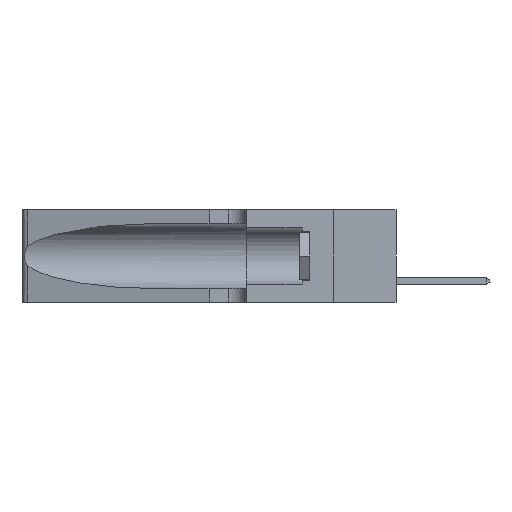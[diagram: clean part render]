
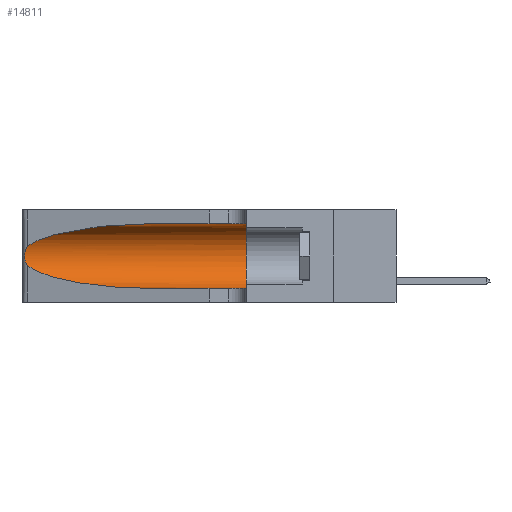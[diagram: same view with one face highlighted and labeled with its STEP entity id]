
A CAD part, left-side view. The second image highlights one B-rep face of the part: STEP entity #14811.
In plain terms, the highlighted cylindrical face has radius 3.308 mm (diameter 6.617 mm), a partial arc.
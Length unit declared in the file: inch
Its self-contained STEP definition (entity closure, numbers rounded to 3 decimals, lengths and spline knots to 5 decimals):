
#454 = EDGE_CURVE ( 'NONE', #9702, #13073, #2145, .T. ) ;
#781 = CARTESIAN_POINT ( 'NONE',  ( 0.1305, 0.72297, 0.31525 ) ) ;
#1479 = CARTESIAN_POINT ( 'NONE',  ( 0.1305, 1.61858, 0.31525 ) ) ;
#2141 = CARTESIAN_POINT ( 'NONE',  ( 0.25856, 1.23593, 0.16098 ) ) ;
#2145 =( BOUNDED_CURVE ( )  B_SPLINE_CURVE ( 3, ( #781, #26645, #13333, #13457 ),
 .UNSPECIFIED., .F., .T. ) 
 B_SPLINE_CURVE_WITH_KNOTS ( ( 4, 4 ),
 ( 1.5708, 2.84003 ),
 .UNSPECIFIED. ) 
 CURVE ( )  GEOMETRIC_REPRESENTATION_ITEM ( )  RATIONAL_B_SPLINE_CURVE ( ( 1., 0.87, 0.87, 1. ) ) 
 REPRESENTATION_ITEM ( '' )  );
#2246 = CARTESIAN_POINT ( 'NONE',  ( 0.25639, 1.23184, 0.21858 ) ) ;
#2332 = B_SPLINE_CURVE_WITH_KNOTS ( 'NONE', 3,
 ( #25720, #20434, #2246, #20649, #7427, #25504, #9921, #10036, #7210, #2141, #9804, #23312, #28381, #4944 ),
 .UNSPECIFIED., .F., .F.,
 ( 4, 2, 2, 2, 2, 2, 4 ),
 ( 0., 0.00027, 0.00053, 0.00107, 0.0016, 0.00187, 0.00214 ),
 .UNSPECIFIED. ) ;
#4106 = VERTEX_POINT ( 'NONE', #18051 ) ;
#4324 = VERTEX_POINT ( 'NONE', #7774 ) ;
#4944 = CARTESIAN_POINT ( 'NONE',  ( 0.25487, 1.22718, 0.14631 ) ) ;
#7031 = ORIENTED_EDGE ( 'NONE', *, *, #20623, .T. ) ;
#7078 = CARTESIAN_POINT ( 'NONE',  ( 0.1305, 1.61858, 0.05475 ) ) ;
#7210 = CARTESIAN_POINT ( 'NONE',  ( 0.26017, 1.23833, 0.17102 ) ) ;
#7427 = CARTESIAN_POINT ( 'NONE',  ( 0.25854, 1.2359, 0.20912 ) ) ;
#7488 = CIRCLE ( 'NONE', #22360, 0.13025 ) ;
#7774 = CARTESIAN_POINT ( 'NONE',  ( 0.25487, 1.22718, 0.14631 ) ) ;
#8549 = VERTEX_POINT ( 'NONE', #9914 ) ;
#9207 = DIRECTION ( 'NONE',  ( 0., -1., 0. ) ) ;
#9702 = VERTEX_POINT ( 'NONE', #19560 ) ;
#9804 = CARTESIAN_POINT ( 'NONE',  ( 0.25789, 1.23486, 0.15765 ) ) ;
#9914 = CARTESIAN_POINT ( 'NONE',  ( 0.1305, 0.35, 0.31525 ) ) ;
#9921 = CARTESIAN_POINT ( 'NONE',  ( 0.26075, 1.23896, 0.19203 ) ) ;
#10036 = CARTESIAN_POINT ( 'NONE',  ( 0.26075, 1.23896, 0.178 ) ) ;
#11297 = ORIENTED_EDGE ( 'NONE', *, *, #27609, .F. ) ;
#11868 = DIRECTION ( 'NONE',  ( 0., -1., 0. ) ) ;
#11977 = VECTOR ( 'NONE', #11868, 39.37008 ) ;
#12317 = EDGE_LOOP ( 'NONE', ( #15542, #32672, #7031, #12323, #17572, #11297 ) ) ;
#12323 = ORIENTED_EDGE ( 'NONE', *, *, #17077, .T. ) ;
#13073 = VERTEX_POINT ( 'NONE', #16088 ) ;
#13234 = FACE_OUTER_BOUND ( 'NONE', #12317, .T. ) ;
#13333 = CARTESIAN_POINT ( 'NONE',  ( 0.2373, 1.15595, 0.28018 ) ) ;
#13457 = CARTESIAN_POINT ( 'NONE',  ( 0.25487, 1.22718, 0.22369 ) ) ;
#14811 = ADVANCED_FACE ( 'NONE', ( #13234 ), #21000, .F. ) ;
#15542 = ORIENTED_EDGE ( 'NONE', *, *, #454, .T. ) ;
#16088 = CARTESIAN_POINT ( 'NONE',  ( 0.25487, 1.22718, 0.22369 ) ) ;
#17077 = EDGE_CURVE ( 'NONE', #33320, #4106, #25706, .T. ) ;
#17572 = ORIENTED_EDGE ( 'NONE', *, *, #29196, .F. ) ;
#18051 = CARTESIAN_POINT ( 'NONE',  ( 0.1305, 0.35, 0.05475 ) ) ;
#19560 = CARTESIAN_POINT ( 'NONE',  ( 0.1305, 0.72297, 0.31525 ) ) ;
#19934 = VECTOR ( 'NONE', #27773, 39.37008 ) ;
#20434 = CARTESIAN_POINT ( 'NONE',  ( 0.25555, 1.22994, 0.2215 ) ) ;
#20623 = EDGE_CURVE ( 'NONE', #4324, #33320, #23007, .T. ) ;
#20649 = CARTESIAN_POINT ( 'NONE',  ( 0.25787, 1.23484, 0.2124 ) ) ;
#20745 = CARTESIAN_POINT ( 'NONE',  ( 0.1305, 0.72297, 0.05475 ) ) ;
#21000 = CYLINDRICAL_SURFACE ( 'NONE', #31091, 0.13025 ) ;
#22360 = AXIS2_PLACEMENT_3D ( 'NONE', #30565, #25264, #33278 ) ;
#22463 = EDGE_CURVE ( 'NONE', #13073, #4324, #2332, .T. ) ;
#23007 =( BOUNDED_CURVE ( )  B_SPLINE_CURVE ( 3, ( #25382, #28132, #23308, #20745 ),
 .UNSPECIFIED., .F., .T. ) 
 B_SPLINE_CURVE_WITH_KNOTS ( ( 4, 4 ),
 ( 3.44316, 4.71239 ),
 .UNSPECIFIED. ) 
 CURVE ( )  GEOMETRIC_REPRESENTATION_ITEM ( )  RATIONAL_B_SPLINE_CURVE ( ( 1., 0.87, 0.87, 1. ) ) 
 REPRESENTATION_ITEM ( '' )  );
#23308 = CARTESIAN_POINT ( 'NONE',  ( 0.18966, 0.96281, 0.05475 ) ) ;
#23312 = CARTESIAN_POINT ( 'NONE',  ( 0.25639, 1.23186, 0.15144 ) ) ;
#25264 = DIRECTION ( 'NONE',  ( 0., 1., 0. ) ) ;
#25382 = CARTESIAN_POINT ( 'NONE',  ( 0.25487, 1.22718, 0.14631 ) ) ;
#25504 = CARTESIAN_POINT ( 'NONE',  ( 0.26018, 1.23835, 0.19895 ) ) ;
#25706 = LINE ( 'NONE', #7078, #19934 ) ;
#25720 = CARTESIAN_POINT ( 'NONE',  ( 0.25487, 1.22718, 0.22369 ) ) ;
#26645 = CARTESIAN_POINT ( 'NONE',  ( 0.18966, 0.96281, 0.31525 ) ) ;
#27301 = CARTESIAN_POINT ( 'NONE',  ( 0.1305, 1.61858, 0.185 ) ) ;
#27609 = EDGE_CURVE ( 'NONE', #9702, #8549, #30033, .T. ) ;
#27645 = DIRECTION ( 'NONE',  ( 0., 0., -1. ) ) ;
#27773 = DIRECTION ( 'NONE',  ( 0., -1., 0. ) ) ;
#28132 = CARTESIAN_POINT ( 'NONE',  ( 0.2373, 1.15595, 0.08982 ) ) ;
#28381 = CARTESIAN_POINT ( 'NONE',  ( 0.25555, 1.22993, 0.14849 ) ) ;
#29196 = EDGE_CURVE ( 'NONE', #8549, #4106, #7488, .T. ) ;
#30033 = LINE ( 'NONE', #1479, #11977 ) ;
#30300 = CARTESIAN_POINT ( 'NONE',  ( 0.1305, 0.72297, 0.05475 ) ) ;
#30565 = CARTESIAN_POINT ( 'NONE',  ( 0.1305, 0.35, 0.185 ) ) ;
#31091 = AXIS2_PLACEMENT_3D ( 'NONE', #27301, #9207, #27645 ) ;
#32672 = ORIENTED_EDGE ( 'NONE', *, *, #22463, .T. ) ;
#33278 = DIRECTION ( 'NONE',  ( 0., 0., 1. ) ) ;
#33320 = VERTEX_POINT ( 'NONE', #30300 ) ;
